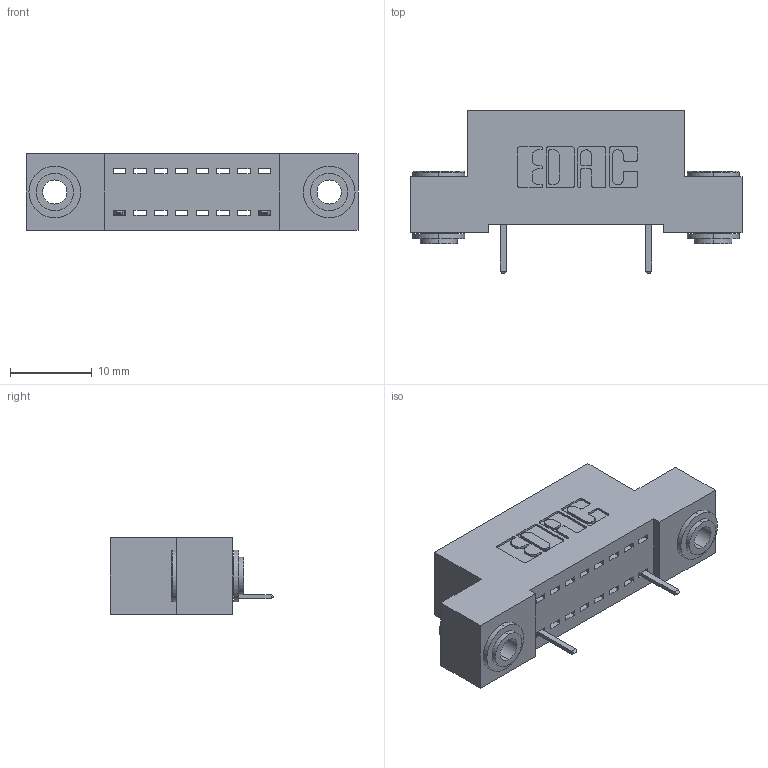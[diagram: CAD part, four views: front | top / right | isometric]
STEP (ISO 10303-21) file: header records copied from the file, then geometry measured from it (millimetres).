
FILE_DESCRIPTION (( 'STEP AP203' ), '1' );
FILE_NAME ('392-008-520-103.STEP', '2018-08-14T19:07:18', ( '' ), ( '' ), 'SwSTEP 2.0', 'SolidWorks 2016', '' );
FILE_SCHEMA (( 'CONFIG_CONTROL_DESIGN' ));
Length unit declared in the file: inch
Products named in the file (4): 342 Part_.156 TH; 345-292-001_345-293-120; 342-250-002_345-250-002-102; 392-008-520-103
Assembly tree (5 placements, depth 2):
  392-008-520-103
    342 Part_.156 TH
    345-292-001_345-293-120  x2
    342-250-002_345-250-002-102  x2
Bounding box: 40.64 x 20.02 x 9.4 mm (x, y, z)
Volume: 3386.5 mm3; surface area: 4190.3 mm2
Topology: 5 solids, 5 shells, 344 faces, 995 edges, 654 vertices
Faces by surface type: plane 236, cylinder 100, cone 8
Entity records: 9728 total; most frequent: CARTESIAN_POINT 1699, ORIENTED_EDGE 1630, DIRECTION 1517, EDGE_CURVE 815, VECTOR 659, LINE 659, VERTEX_POINT 538, AXIS2_PLACEMENT_3D 429
